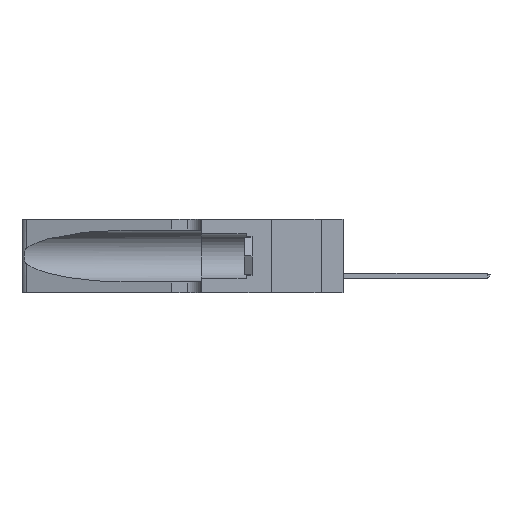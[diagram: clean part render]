
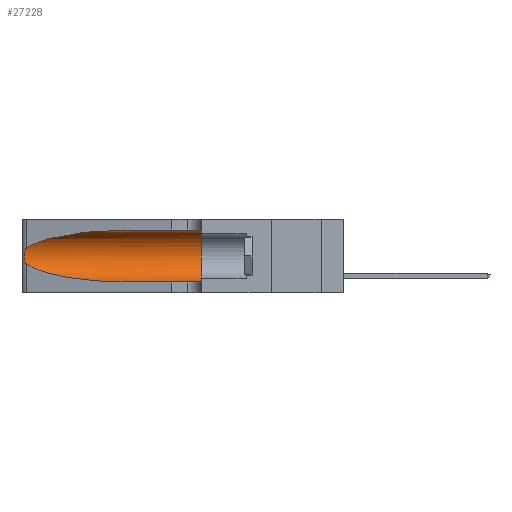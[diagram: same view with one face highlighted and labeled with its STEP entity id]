
A CAD part, left-side view. The second image highlights one B-rep face of the part: STEP entity #27228.
In plain terms, the highlighted cylindrical face has radius 3.308 mm (diameter 6.617 mm), a partial arc.
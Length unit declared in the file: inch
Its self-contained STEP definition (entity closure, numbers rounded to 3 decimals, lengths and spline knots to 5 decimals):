
#296 = CARTESIAN_POINT ( 'NONE',  ( 0.25487, 1.22718, 0.22369 ) ) ;
#3137 = FACE_OUTER_BOUND ( 'NONE', #38172, .T. ) ;
#4605 = CARTESIAN_POINT ( 'NONE',  ( 0.1305, 1.61858, 0.31525 ) ) ;
#4799 = B_SPLINE_CURVE_WITH_KNOTS ( 'NONE', 3,
 ( #28143, #43172, #24557, #32400, #5651, #31889, #28638, #9406, #5816, #32068, #9903, #36142, #13700, #17503 ),
 .UNSPECIFIED., .F., .F.,
 ( 4, 2, 2, 2, 2, 2, 4 ),
 ( 0., 0.00027, 0.00053, 0.00107, 0.0016, 0.00187, 0.00214 ),
 .UNSPECIFIED. ) ;
#5651 = CARTESIAN_POINT ( 'NONE',  ( 0.25854, 1.2359, 0.20912 ) ) ;
#5772 = VERTEX_POINT ( 'NONE', #6732 ) ;
#5816 = CARTESIAN_POINT ( 'NONE',  ( 0.26017, 1.23833, 0.17102 ) ) ;
#6732 = CARTESIAN_POINT ( 'NONE',  ( 0.1305, 0.72297, 0.05475 ) ) ;
#6744 = ORIENTED_EDGE ( 'NONE', *, *, #11274, .T. ) ;
#6747 = ORIENTED_EDGE ( 'NONE', *, *, #31900, .F. ) ;
#7143 = CARTESIAN_POINT ( 'NONE',  ( 0.1305, 0.35, 0.05475 ) ) ;
#7193 = VERTEX_POINT ( 'NONE', #9522 ) ;
#7299 = CARTESIAN_POINT ( 'NONE',  ( 0.25487, 1.22718, 0.22369 ) ) ;
#7395 = CARTESIAN_POINT ( 'NONE',  ( 0.25487, 1.22718, 0.14631 ) ) ;
#7859 = VERTEX_POINT ( 'NONE', #7143 ) ;
#8378 = DIRECTION ( 'NONE',  ( 0., 0., 1. ) ) ;
#8872 = EDGE_CURVE ( 'NONE', #26162, #37793, #13598, .T. ) ;
#9406 = CARTESIAN_POINT ( 'NONE',  ( 0.26075, 1.23896, 0.178 ) ) ;
#9522 = CARTESIAN_POINT ( 'NONE',  ( 0.25487, 1.22718, 0.14631 ) ) ;
#9903 = CARTESIAN_POINT ( 'NONE',  ( 0.25789, 1.23486, 0.15765 ) ) ;
#9964 = VECTOR ( 'NONE', #38852, 39.37008 ) ;
#11274 = EDGE_CURVE ( 'NONE', #37793, #7193, #4799, .T. ) ;
#12318 = DIRECTION ( 'NONE',  ( 0., 1., 0. ) ) ;
#12508 = ORIENTED_EDGE ( 'NONE', *, *, #21889, .T. ) ;
#13598 =( BOUNDED_CURVE ( )  B_SPLINE_CURVE ( 3, ( #19145, #37439, #19306, #7299 ),
 .UNSPECIFIED., .F., .T. ) 
 B_SPLINE_CURVE_WITH_KNOTS ( ( 4, 4 ),
 ( 1.5708, 2.84003 ),
 .UNSPECIFIED. ) 
 CURVE ( )  GEOMETRIC_REPRESENTATION_ITEM ( )  RATIONAL_B_SPLINE_CURVE ( ( 1., 0.87, 0.87, 1. ) ) 
 REPRESENTATION_ITEM ( '' )  );
#13700 = CARTESIAN_POINT ( 'NONE',  ( 0.25555, 1.22993, 0.14849 ) ) ;
#13815 = CARTESIAN_POINT ( 'NONE',  ( 0.2373, 1.15595, 0.08982 ) ) ;
#13820 = VECTOR ( 'NONE', #34495, 39.37008 ) ;
#17503 = CARTESIAN_POINT ( 'NONE',  ( 0.25487, 1.22718, 0.14631 ) ) ;
#17794 = ORIENTED_EDGE ( 'NONE', *, *, #33207, .T. ) ;
#17965 = AXIS2_PLACEMENT_3D ( 'NONE', #38681, #12318, #8378 ) ;
#19145 = CARTESIAN_POINT ( 'NONE',  ( 0.1305, 0.72297, 0.31525 ) ) ;
#19306 = CARTESIAN_POINT ( 'NONE',  ( 0.2373, 1.15595, 0.28018 ) ) ;
#19699 = CARTESIAN_POINT ( 'NONE',  ( 0.1305, 0.72297, 0.05475 ) ) ;
#21889 = EDGE_CURVE ( 'NONE', #5772, #7859, #44594, .T. ) ;
#24289 = CYLINDRICAL_SURFACE ( 'NONE', #31365, 0.13025 ) ;
#24557 = CARTESIAN_POINT ( 'NONE',  ( 0.25639, 1.23184, 0.21858 ) ) ;
#26162 = VERTEX_POINT ( 'NONE', #38470 ) ;
#26221 = ORIENTED_EDGE ( 'NONE', *, *, #41912, .F. ) ;
#26689 = LINE ( 'NONE', #4605, #13820 ) ;
#27228 = ADVANCED_FACE ( 'NONE', ( #3137 ), #24289, .F. ) ;
#28143 = CARTESIAN_POINT ( 'NONE',  ( 0.25487, 1.22718, 0.22369 ) ) ;
#28638 = CARTESIAN_POINT ( 'NONE',  ( 0.26075, 1.23896, 0.19203 ) ) ;
#30174 = VERTEX_POINT ( 'NONE', #48055 ) ;
#30345 = CARTESIAN_POINT ( 'NONE',  ( 0.18966, 0.96281, 0.05475 ) ) ;
#30940 = CARTESIAN_POINT ( 'NONE',  ( 0.1305, 1.61858, 0.05475 ) ) ;
#31365 = AXIS2_PLACEMENT_3D ( 'NONE', #34898, #34585, #41911 ) ;
#31889 = CARTESIAN_POINT ( 'NONE',  ( 0.26018, 1.23835, 0.19895 ) ) ;
#31900 = EDGE_CURVE ( 'NONE', #26162, #30174, #26689, .T. ) ;
#32068 = CARTESIAN_POINT ( 'NONE',  ( 0.25856, 1.23593, 0.16098 ) ) ;
#32203 = ORIENTED_EDGE ( 'NONE', *, *, #8872, .T. ) ;
#32400 = CARTESIAN_POINT ( 'NONE',  ( 0.25787, 1.23484, 0.2124 ) ) ;
#33207 = EDGE_CURVE ( 'NONE', #7193, #5772, #39062, .T. ) ;
#34495 = DIRECTION ( 'NONE',  ( 0., -1., 0. ) ) ;
#34585 = DIRECTION ( 'NONE',  ( 0., -1., 0. ) ) ;
#34898 = CARTESIAN_POINT ( 'NONE',  ( 0.1305, 1.61858, 0.185 ) ) ;
#36142 = CARTESIAN_POINT ( 'NONE',  ( 0.25639, 1.23186, 0.15144 ) ) ;
#37439 = CARTESIAN_POINT ( 'NONE',  ( 0.18966, 0.96281, 0.31525 ) ) ;
#37793 = VERTEX_POINT ( 'NONE', #296 ) ;
#38172 = EDGE_LOOP ( 'NONE', ( #32203, #6744, #17794, #12508, #26221, #6747 ) ) ;
#38470 = CARTESIAN_POINT ( 'NONE',  ( 0.1305, 0.72297, 0.31525 ) ) ;
#38681 = CARTESIAN_POINT ( 'NONE',  ( 0.1305, 0.35, 0.185 ) ) ;
#38852 = DIRECTION ( 'NONE',  ( 0., -1., 0. ) ) ;
#38962 = CIRCLE ( 'NONE', #17965, 0.13025 ) ;
#39062 =( BOUNDED_CURVE ( )  B_SPLINE_CURVE ( 3, ( #7395, #13815, #30345, #19699 ),
 .UNSPECIFIED., .F., .T. ) 
 B_SPLINE_CURVE_WITH_KNOTS ( ( 4, 4 ),
 ( 3.44316, 4.71239 ),
 .UNSPECIFIED. ) 
 CURVE ( )  GEOMETRIC_REPRESENTATION_ITEM ( )  RATIONAL_B_SPLINE_CURVE ( ( 1., 0.87, 0.87, 1. ) ) 
 REPRESENTATION_ITEM ( '' )  );
#41911 = DIRECTION ( 'NONE',  ( 0., 0., -1. ) ) ;
#41912 = EDGE_CURVE ( 'NONE', #30174, #7859, #38962, .T. ) ;
#43172 = CARTESIAN_POINT ( 'NONE',  ( 0.25555, 1.22994, 0.2215 ) ) ;
#44594 = LINE ( 'NONE', #30940, #9964 ) ;
#48055 = CARTESIAN_POINT ( 'NONE',  ( 0.1305, 0.35, 0.31525 ) ) ;
